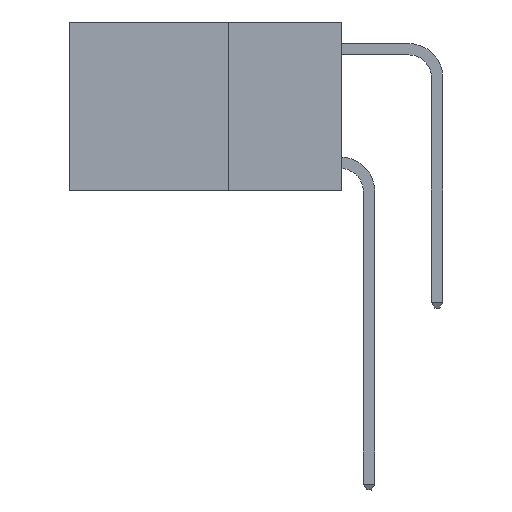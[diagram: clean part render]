
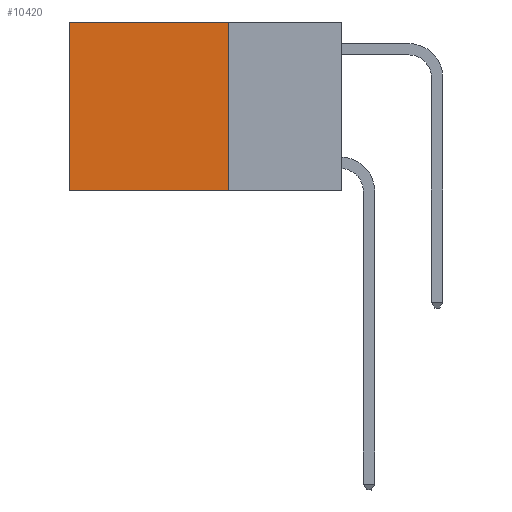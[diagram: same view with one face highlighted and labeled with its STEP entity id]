
A CAD part, left-side view. The second image highlights one B-rep face of the part: STEP entity #10420.
In plain terms, the highlighted planar face has unit normal (-1, 0, 0).
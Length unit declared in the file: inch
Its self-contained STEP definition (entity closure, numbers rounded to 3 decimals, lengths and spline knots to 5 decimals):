
#794 = VECTOR ( 'NONE', #11818, 39.37008 ) ;
#833 = DIRECTION ( 'NONE',  ( 0., 0., -1. ) ) ;
#875 = FACE_OUTER_BOUND ( 'NONE', #11162, .T. ) ;
#1097 = VERTEX_POINT ( 'NONE', #19154 ) ;
#1558 = VECTOR ( 'NONE', #4124, 39.37008 ) ;
#1689 = CARTESIAN_POINT ( 'NONE',  ( 0.2625, 0.25, 0. ) ) ;
#2192 = EDGE_CURVE ( 'NONE', #4454, #16639, #10695, .T. ) ;
#2326 = DIRECTION ( 'NONE',  ( 0., 1., 0. ) ) ;
#2657 = ORIENTED_EDGE ( 'NONE', *, *, #2192, .T. ) ;
#3198 = ORIENTED_EDGE ( 'NONE', *, *, #12137, .F. ) ;
#3911 = LINE ( 'NONE', #5274, #20246 ) ;
#4124 = DIRECTION ( 'NONE',  ( 0., 0., -1. ) ) ;
#4454 = VERTEX_POINT ( 'NONE', #5082 ) ;
#4637 = AXIS2_PLACEMENT_3D ( 'NONE', #19889, #10537, #833 ) ;
#4913 = ORIENTED_EDGE ( 'NONE', *, *, #18112, .T. ) ;
#5082 = CARTESIAN_POINT ( 'NONE',  ( 0.2625, 0.6, 0. ) ) ;
#5274 = CARTESIAN_POINT ( 'NONE',  ( 0.2625, 0.25, -0.37 ) ) ;
#5361 = CARTESIAN_POINT ( 'NONE',  ( 0.2625, 0.25, 0. ) ) ;
#5591 = LINE ( 'NONE', #5361, #794 ) ;
#5899 = VECTOR ( 'NONE', #2326, 39.37008 ) ;
#10420 = ADVANCED_FACE ( 'NONE', ( #875 ), #12099, .F. ) ;
#10537 = DIRECTION ( 'NONE',  ( 1., 0., 0. ) ) ;
#10695 = LINE ( 'NONE', #15399, #1558 ) ;
#10730 = EDGE_CURVE ( 'NONE', #1097, #16639, #3911, .T. ) ;
#10735 = LINE ( 'NONE', #12101, #5899 ) ;
#11162 = EDGE_LOOP ( 'NONE', ( #2657, #12627, #3198, #4913 ) ) ;
#11818 = DIRECTION ( 'NONE',  ( 0., 0., -1. ) ) ;
#11955 = VERTEX_POINT ( 'NONE', #1689 ) ;
#12099 = PLANE ( 'NONE',  #4637 ) ;
#12101 = CARTESIAN_POINT ( 'NONE',  ( 0.2625, 0.25, 0. ) ) ;
#12137 = EDGE_CURVE ( 'NONE', #11955, #1097, #5591, .T. ) ;
#12627 = ORIENTED_EDGE ( 'NONE', *, *, #10730, .F. ) ;
#15399 = CARTESIAN_POINT ( 'NONE',  ( 0.2625, 0.6, 0. ) ) ;
#16530 = DIRECTION ( 'NONE',  ( 0., 1., 0. ) ) ;
#16639 = VERTEX_POINT ( 'NONE', #20247 ) ;
#18112 = EDGE_CURVE ( 'NONE', #11955, #4454, #10735, .T. ) ;
#19154 = CARTESIAN_POINT ( 'NONE',  ( 0.2625, 0.25, -0.37 ) ) ;
#19889 = CARTESIAN_POINT ( 'NONE',  ( 0.2625, 0.25, 0. ) ) ;
#20246 = VECTOR ( 'NONE', #16530, 39.37008 ) ;
#20247 = CARTESIAN_POINT ( 'NONE',  ( 0.2625, 0.6, -0.37 ) ) ;
